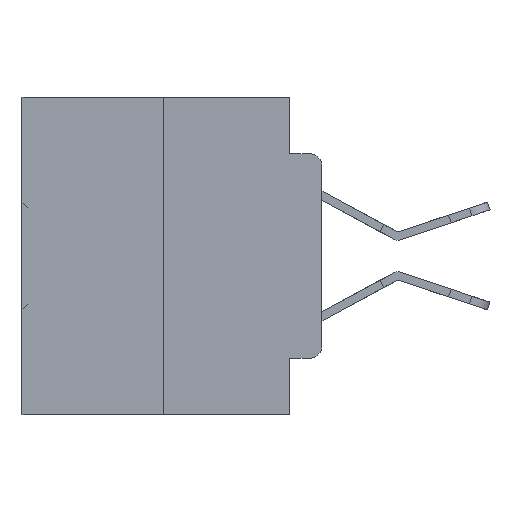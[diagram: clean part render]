
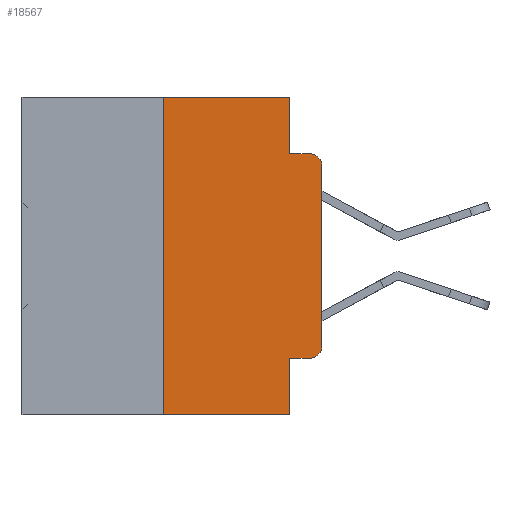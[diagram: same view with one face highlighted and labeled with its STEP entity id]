
A CAD part, left-side view. The second image highlights one B-rep face of the part: STEP entity #18567.
In plain terms, the highlighted planar face has unit normal (-1, 0, 0).
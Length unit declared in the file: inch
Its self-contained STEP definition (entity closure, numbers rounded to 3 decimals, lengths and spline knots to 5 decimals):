
#213 = EDGE_CURVE ( 'NONE', #30351, #10370, #18866, .T. ) ;
#511 = EDGE_CURVE ( 'NONE', #28002, #31069, #20999, .T. ) ;
#725 = CARTESIAN_POINT ( 'NONE',  ( 0., 0.02, -0.3915 ) ) ;
#1313 = EDGE_CURVE ( 'NONE', #31069, #29841, #21885, .T. ) ;
#2281 = DIRECTION ( 'NONE',  ( 0., -1., 0. ) ) ;
#2391 = DIRECTION ( 'NONE',  ( 1., 0., 0. ) ) ;
#3090 = CARTESIAN_POINT ( 'NONE',  ( 0., 0.051, 0. ) ) ;
#3759 = ORIENTED_EDGE ( 'NONE', *, *, #11599, .T. ) ;
#5158 = VECTOR ( 'NONE', #8224, 39.37008 ) ;
#5223 = DIRECTION ( 'NONE',  ( 0., 0., -1. ) ) ;
#5769 = LINE ( 'NONE', #17562, #29071 ) ;
#6099 = CARTESIAN_POINT ( 'NONE',  ( 0., 0., -0.3915 ) ) ;
#6177 = CARTESIAN_POINT ( 'NONE',  ( 0., 0.473, -0.5 ) ) ;
#6355 = CIRCLE ( 'NONE', #29428, 0.02 ) ;
#6685 = EDGE_CURVE ( 'NONE', #12483, #11769, #34751, .T. ) ;
#7293 = DIRECTION ( 'NONE',  ( 0., 0., -1. ) ) ;
#8171 = CARTESIAN_POINT ( 'NONE',  ( 0., 0.051, -0.4115 ) ) ;
#8224 = DIRECTION ( 'NONE',  ( 0., -1., 0. ) ) ;
#8714 = EDGE_CURVE ( 'NONE', #36092, #28002, #35330, .T. ) ;
#9319 = DIRECTION ( 'NONE',  ( 0., 0., 1. ) ) ;
#9442 = ORIENTED_EDGE ( 'NONE', *, *, #511, .F. ) ;
#9943 = CARTESIAN_POINT ( 'NONE',  ( 0., 0., 0. ) ) ;
#10355 = EDGE_CURVE ( 'NONE', #11769, #29841, #28422, .T. ) ;
#10370 = VERTEX_POINT ( 'NONE', #34231 ) ;
#10507 = VECTOR ( 'NONE', #2281, 39.37008 ) ;
#10994 = CARTESIAN_POINT ( 'NONE',  ( 0., 0.473, 0. ) ) ;
#11599 = EDGE_CURVE ( 'NONE', #10370, #12483, #6355, .T. ) ;
#11769 = VERTEX_POINT ( 'NONE', #27050 ) ;
#12215 = VECTOR ( 'NONE', #7293, 39.37008 ) ;
#12483 = VERTEX_POINT ( 'NONE', #6099 ) ;
#13100 = ORIENTED_EDGE ( 'NONE', *, *, #213, .T. ) ;
#13170 = CARTESIAN_POINT ( 'NONE',  ( 0., 0.25, 0. ) ) ;
#13597 = ORIENTED_EDGE ( 'NONE', *, *, #10355, .T. ) ;
#14574 = DIRECTION ( 'NONE',  ( 0., 0., -1. ) ) ;
#15063 = AXIS2_PLACEMENT_3D ( 'NONE', #25764, #25296, #14574 ) ;
#17427 = AXIS2_PLACEMENT_3D ( 'NONE', #10994, #2391, #5223 ) ;
#17562 = CARTESIAN_POINT ( 'NONE',  ( 0., 0.25, 0. ) ) ;
#18034 = VECTOR ( 'NONE', #21836, 39.37008 ) ;
#18392 = ORIENTED_EDGE ( 'NONE', *, *, #19113, .F. ) ;
#18567 = ADVANCED_FACE ( 'NONE', ( #31241 ), #36154, .F. ) ;
#18839 = ORIENTED_EDGE ( 'NONE', *, *, #1313, .F. ) ;
#18866 = LINE ( 'NONE', #33509, #10507 ) ;
#18900 = ORIENTED_EDGE ( 'NONE', *, *, #6685, .T. ) ;
#19113 = EDGE_CURVE ( 'NONE', #33035, #36092, #5769, .T. ) ;
#20003 = ORIENTED_EDGE ( 'NONE', *, *, #8714, .F. ) ;
#20391 = DIRECTION ( 'NONE',  ( -1., 0., 0. ) ) ;
#20999 = LINE ( 'NONE', #24156, #12215 ) ;
#21142 = VERTEX_POINT ( 'NONE', #21984 ) ;
#21836 = DIRECTION ( 'NONE',  ( 0., 0., -1. ) ) ;
#21885 = LINE ( 'NONE', #30606, #5158 ) ;
#21984 = CARTESIAN_POINT ( 'NONE',  ( 0., 0.051, -0.5 ) ) ;
#22094 = LINE ( 'NONE', #6177, #35225 ) ;
#23083 = VECTOR ( 'NONE', #34761, 39.37008 ) ;
#23217 = CARTESIAN_POINT ( 'NONE',  ( 0., 0.051, -0.0885 ) ) ;
#23337 = VECTOR ( 'NONE', #32717, 39.37008 ) ;
#23384 = EDGE_CURVE ( 'NONE', #33035, #21142, #22094, .T. ) ;
#24054 = ORIENTED_EDGE ( 'NONE', *, *, #23384, .T. ) ;
#24156 = CARTESIAN_POINT ( 'NONE',  ( 0., 0.051, 0. ) ) ;
#25296 = DIRECTION ( 'NONE',  ( -1., 0., 0. ) ) ;
#25554 = LINE ( 'NONE', #27132, #18034 ) ;
#25655 = EDGE_LOOP ( 'NONE', ( #18900, #13597, #18839, #9442, #20003, #18392, #24054, #29251, #13100, #3759 ) ) ;
#25764 = CARTESIAN_POINT ( 'NONE',  ( 0., 0.02, -0.1085 ) ) ;
#26132 = CARTESIAN_POINT ( 'NONE',  ( 0., 0.02, -0.0885 ) ) ;
#26221 = DIRECTION ( 'NONE',  ( 0., -1., 0. ) ) ;
#27050 = CARTESIAN_POINT ( 'NONE',  ( 0., 0., -0.1085 ) ) ;
#27132 = CARTESIAN_POINT ( 'NONE',  ( 0., 0.051, 0. ) ) ;
#28002 = VERTEX_POINT ( 'NONE', #3090 ) ;
#28422 = CIRCLE ( 'NONE', #15063, 0.02 ) ;
#29071 = VECTOR ( 'NONE', #9319, 39.37008 ) ;
#29251 = ORIENTED_EDGE ( 'NONE', *, *, #31948, .F. ) ;
#29428 = AXIS2_PLACEMENT_3D ( 'NONE', #725, #20391, #34294 ) ;
#29841 = VERTEX_POINT ( 'NONE', #26132 ) ;
#30351 = VERTEX_POINT ( 'NONE', #8171 ) ;
#30606 = CARTESIAN_POINT ( 'NONE',  ( 0., 0.051, -0.0885 ) ) ;
#31069 = VERTEX_POINT ( 'NONE', #23217 ) ;
#31241 = FACE_OUTER_BOUND ( 'NONE', #25655, .T. ) ;
#31948 = EDGE_CURVE ( 'NONE', #30351, #21142, #25554, .T. ) ;
#31960 = CARTESIAN_POINT ( 'NONE',  ( 0., 0.473, 0. ) ) ;
#32717 = DIRECTION ( 'NONE',  ( 0., 0., 1. ) ) ;
#33035 = VERTEX_POINT ( 'NONE', #36304 ) ;
#33509 = CARTESIAN_POINT ( 'NONE',  ( 0., 0.051, -0.4115 ) ) ;
#34231 = CARTESIAN_POINT ( 'NONE',  ( 0., 0.02, -0.4115 ) ) ;
#34294 = DIRECTION ( 'NONE',  ( 0., 0., -1. ) ) ;
#34751 = LINE ( 'NONE', #9943, #23337 ) ;
#34761 = DIRECTION ( 'NONE',  ( 0., -1., 0. ) ) ;
#35225 = VECTOR ( 'NONE', #26221, 39.37008 ) ;
#35330 = LINE ( 'NONE', #31960, #23083 ) ;
#36092 = VERTEX_POINT ( 'NONE', #13170 ) ;
#36154 = PLANE ( 'NONE',  #17427 ) ;
#36304 = CARTESIAN_POINT ( 'NONE',  ( 0., 0.25, -0.5 ) ) ;
